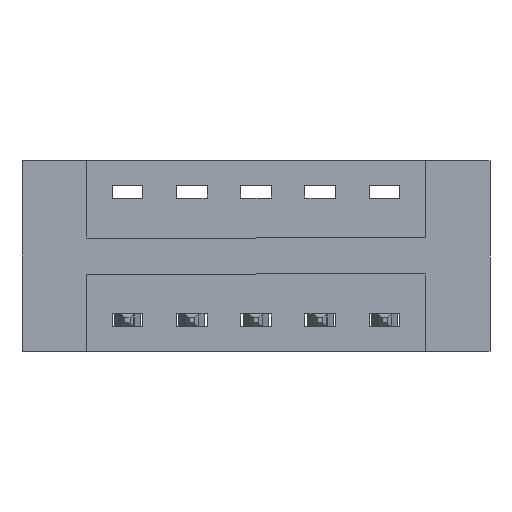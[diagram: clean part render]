
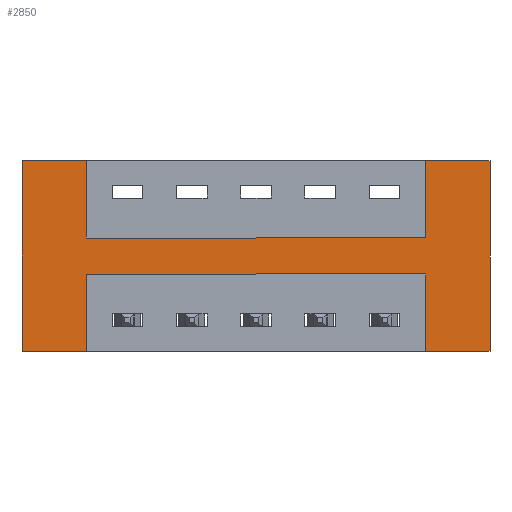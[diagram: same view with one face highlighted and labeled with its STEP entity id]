
A CAD part, front view. The second image highlights one B-rep face of the part: STEP entity #2850.
In plain terms, the highlighted planar face has unit normal (0, -1, 0).
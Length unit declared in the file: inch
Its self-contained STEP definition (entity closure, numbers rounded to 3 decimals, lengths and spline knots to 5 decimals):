
#31 = CARTESIAN_POINT ( 'NONE',  ( 0.3875, 0., -0.22 ) ) ;
#55 = VECTOR ( 'NONE', #2207, 39.37008 ) ;
#61 = CARTESIAN_POINT ( 'NONE',  ( 1.0475, 0., -0.15 ) ) ;
#148 = VECTOR ( 'NONE', #6902, 39.37008 ) ;
#377 = LINE ( 'NONE', #5680, #2736 ) ;
#515 = VERTEX_POINT ( 'NONE', #6530 ) ;
#652 = EDGE_CURVE ( 'NONE', #2131, #5059, #6831, .T. ) ;
#659 = FACE_OUTER_BOUND ( 'NONE', #7509, .T. ) ;
#681 = DIRECTION ( 'NONE',  ( 0., 0., -1. ) ) ;
#723 = EDGE_CURVE ( 'NONE', #7741, #4933, #3118, .T. ) ;
#871 = ORIENTED_EDGE ( 'NONE', *, *, #3065, .F. ) ;
#885 = VECTOR ( 'NONE', #1560, 39.37008 ) ;
#896 = EDGE_CURVE ( 'NONE', #1618, #3155, #3788, .T. ) ;
#932 = EDGE_CURVE ( 'NONE', #2131, #515, #377, .T. ) ;
#978 = VERTEX_POINT ( 'NONE', #4905 ) ;
#1037 = VERTEX_POINT ( 'NONE', #6495 ) ;
#1042 = VERTEX_POINT ( 'NONE', #31 ) ;
#1155 = ORIENTED_EDGE ( 'NONE', *, *, #7842, .F. ) ;
#1356 = EDGE_CURVE ( 'NONE', #1042, #7829, #3111, .T. ) ;
#1420 = VECTOR ( 'NONE', #4135, 39.37008 ) ;
#1560 = DIRECTION ( 'NONE',  ( -1., 0., 0. ) ) ;
#1618 = VERTEX_POINT ( 'NONE', #7739 ) ;
#1726 = DIRECTION ( 'NONE',  ( 0., -1., 0. ) ) ;
#1748 = DIRECTION ( 'NONE',  ( -1., 0., 0. ) ) ;
#1805 = ORIENTED_EDGE ( 'NONE', *, *, #1356, .F. ) ;
#2027 = ORIENTED_EDGE ( 'NONE', *, *, #2084, .F. ) ;
#2084 = EDGE_CURVE ( 'NONE', #978, #5072, #6562, .T. ) ;
#2131 = VERTEX_POINT ( 'NONE', #7713 ) ;
#2133 = VECTOR ( 'NONE', #6662, 39.37008 ) ;
#2207 = DIRECTION ( 'NONE',  ( 0., 0., -1. ) ) ;
#2381 = CARTESIAN_POINT ( 'NONE',  ( 0., 0., 0. ) ) ;
#2477 = DIRECTION ( 'NONE',  ( 1., 0., 0. ) ) ;
#2579 = VECTOR ( 'NONE', #5250, 39.37008 ) ;
#2631 = ORIENTED_EDGE ( 'NONE', *, *, #3981, .F. ) ;
#2736 = VECTOR ( 'NONE', #2477, 39.37008 ) ;
#2850 = ADVANCED_FACE ( 'NONE', ( #659 ), #4400, .T. ) ;
#2971 = ORIENTED_EDGE ( 'NONE', *, *, #932, .F. ) ;
#3048 = CARTESIAN_POINT ( 'NONE',  ( 0.3875, 0., -0.15 ) ) ;
#3065 = EDGE_CURVE ( 'NONE', #4933, #1042, #6038, .T. ) ;
#3066 = CARTESIAN_POINT ( 'NONE',  ( 0.3875, 0., -0.37 ) ) ;
#3100 = LINE ( 'NONE', #6494, #1420 ) ;
#3111 = LINE ( 'NONE', #5486, #7547 ) ;
#3118 = LINE ( 'NONE', #7620, #6317 ) ;
#3155 = VERTEX_POINT ( 'NONE', #61 ) ;
#3394 = CARTESIAN_POINT ( 'NONE',  ( 0.3875, 0., -0.22 ) ) ;
#3532 = AXIS2_PLACEMENT_3D ( 'NONE', #5462, #1726, #4353 ) ;
#3717 = ORIENTED_EDGE ( 'NONE', *, *, #896, .F. ) ;
#3788 = LINE ( 'NONE', #3048, #2133 ) ;
#3890 = EDGE_CURVE ( 'NONE', #1037, #7741, #6980, .T. ) ;
#3981 = EDGE_CURVE ( 'NONE', #7829, #5059, #3100, .T. ) ;
#4009 = VECTOR ( 'NONE', #7167, 39.37008 ) ;
#4043 = CARTESIAN_POINT ( 'NONE',  ( 1.0475, 0., -0.22 ) ) ;
#4135 = DIRECTION ( 'NONE',  ( -1., 0., 0. ) ) ;
#4158 = ORIENTED_EDGE ( 'NONE', *, *, #6056, .T. ) ;
#4212 = LINE ( 'NONE', #6924, #2579 ) ;
#4295 = CARTESIAN_POINT ( 'NONE',  ( 1.0475, 0., 0. ) ) ;
#4353 = DIRECTION ( 'NONE',  ( 0., 0., -1. ) ) ;
#4400 = PLANE ( 'NONE',  #3532 ) ;
#4574 = CARTESIAN_POINT ( 'NONE',  ( 1.1725, 0., 0. ) ) ;
#4734 = ORIENTED_EDGE ( 'NONE', *, *, #652, .T. ) ;
#4905 = CARTESIAN_POINT ( 'NONE',  ( 1.0475, 0., 0. ) ) ;
#4933 = VERTEX_POINT ( 'NONE', #4043 ) ;
#4975 = DIRECTION ( 'NONE',  ( 0., 0., 1. ) ) ;
#5005 = ORIENTED_EDGE ( 'NONE', *, *, #3890, .F. ) ;
#5059 = VERTEX_POINT ( 'NONE', #5433 ) ;
#5072 = VERTEX_POINT ( 'NONE', #6023 ) ;
#5151 = CARTESIAN_POINT ( 'NONE',  ( 0.2625, 0., 0. ) ) ;
#5250 = DIRECTION ( 'NONE',  ( 0., 0., -1. ) ) ;
#5381 = VECTOR ( 'NONE', #4975, 39.37008 ) ;
#5433 = CARTESIAN_POINT ( 'NONE',  ( 0.2625, 0., -0.37 ) ) ;
#5462 = CARTESIAN_POINT ( 'NONE',  ( 0., 0., -0.37 ) ) ;
#5486 = CARTESIAN_POINT ( 'NONE',  ( 0.3875, 0., -0.37 ) ) ;
#5491 = DIRECTION ( 'NONE',  ( 0., 0., 1. ) ) ;
#5680 = CARTESIAN_POINT ( 'NONE',  ( 0., 0., 0. ) ) ;
#5813 = LINE ( 'NONE', #4295, #4009 ) ;
#6023 = CARTESIAN_POINT ( 'NONE',  ( 1.1725, 0., 0. ) ) ;
#6038 = LINE ( 'NONE', #3394, #7618 ) ;
#6056 = EDGE_CURVE ( 'NONE', #1037, #5072, #6878, .T. ) ;
#6317 = VECTOR ( 'NONE', #5491, 39.37008 ) ;
#6493 = ORIENTED_EDGE ( 'NONE', *, *, #7009, .F. ) ;
#6494 = CARTESIAN_POINT ( 'NONE',  ( 0., 0., -0.37 ) ) ;
#6495 = CARTESIAN_POINT ( 'NONE',  ( 1.1725, 0., -0.37 ) ) ;
#6530 = CARTESIAN_POINT ( 'NONE',  ( 0.3875, 0., 0. ) ) ;
#6562 = LINE ( 'NONE', #2381, #148 ) ;
#6662 = DIRECTION ( 'NONE',  ( 1., 0., 0. ) ) ;
#6714 = ORIENTED_EDGE ( 'NONE', *, *, #723, .F. ) ;
#6831 = LINE ( 'NONE', #5151, #55 ) ;
#6878 = LINE ( 'NONE', #4574, #5381 ) ;
#6902 = DIRECTION ( 'NONE',  ( 1., 0., 0. ) ) ;
#6924 = CARTESIAN_POINT ( 'NONE',  ( 0.3875, 0., 0. ) ) ;
#6980 = LINE ( 'NONE', #6988, #885 ) ;
#6988 = CARTESIAN_POINT ( 'NONE',  ( 0., 0., -0.37 ) ) ;
#7009 = EDGE_CURVE ( 'NONE', #515, #1618, #4212, .T. ) ;
#7096 = CARTESIAN_POINT ( 'NONE',  ( 1.0475, 0., -0.37 ) ) ;
#7167 = DIRECTION ( 'NONE',  ( 0., 0., 1. ) ) ;
#7509 = EDGE_LOOP ( 'NONE', ( #4158, #2027, #1155, #3717, #6493, #2971, #4734, #2631, #1805, #871, #6714, #5005 ) ) ;
#7547 = VECTOR ( 'NONE', #681, 39.37008 ) ;
#7618 = VECTOR ( 'NONE', #1748, 39.37008 ) ;
#7620 = CARTESIAN_POINT ( 'NONE',  ( 1.0475, 0., -0.37 ) ) ;
#7713 = CARTESIAN_POINT ( 'NONE',  ( 0.2625, 0., 0. ) ) ;
#7739 = CARTESIAN_POINT ( 'NONE',  ( 0.3875, 0., -0.15 ) ) ;
#7741 = VERTEX_POINT ( 'NONE', #7096 ) ;
#7829 = VERTEX_POINT ( 'NONE', #3066 ) ;
#7842 = EDGE_CURVE ( 'NONE', #3155, #978, #5813, .T. ) ;
